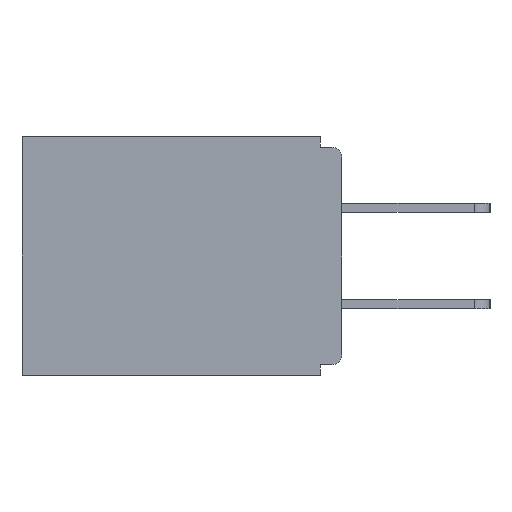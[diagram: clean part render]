
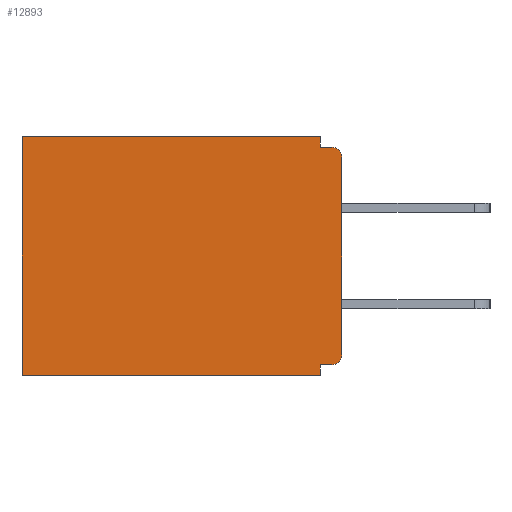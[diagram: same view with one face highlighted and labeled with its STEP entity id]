
A CAD part, left-side view. The second image highlights one B-rep face of the part: STEP entity #12893.
In plain terms, the highlighted planar face has unit normal (-1, 0, 0).
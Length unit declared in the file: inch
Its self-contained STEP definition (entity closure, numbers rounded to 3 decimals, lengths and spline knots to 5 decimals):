
#39 = LINE ( 'NONE', #16850, #4491 ) ;
#577 = EDGE_LOOP ( 'NONE', ( #16964, #21530, #7711, #17324, #13636, #9367, #11349, #9855, #5133, #16486 ) ) ;
#677 = VECTOR ( 'NONE', #12120, 39.37008 ) ;
#1747 = CARTESIAN_POINT ( 'NONE',  ( 0.298, 0., -0.343 ) ) ;
#2031 = DIRECTION ( 'NONE',  ( 0., 0., -1. ) ) ;
#3687 = DIRECTION ( 'NONE',  ( -1., 0., 0. ) ) ;
#3743 = DIRECTION ( 'NONE',  ( 0., 1., 0. ) ) ;
#4325 = LINE ( 'NONE', #12921, #9213 ) ;
#4491 = VECTOR ( 'NONE', #19099, 39.37008 ) ;
#4637 = CARTESIAN_POINT ( 'NONE',  ( 0.298, 0.46, 0. ) ) ;
#5065 = VERTEX_POINT ( 'NONE', #9523 ) ;
#5075 = DIRECTION ( 'NONE',  ( 0., 0., -1. ) ) ;
#5133 = ORIENTED_EDGE ( 'NONE', *, *, #8164, .T. ) ;
#5738 = CARTESIAN_POINT ( 'NONE',  ( 0.298, 0., 0. ) ) ;
#5801 = VERTEX_POINT ( 'NONE', #16505 ) ;
#6765 = DIRECTION ( 'NONE',  ( 0., 0., -1. ) ) ;
#6874 = AXIS2_PLACEMENT_3D ( 'NONE', #23758, #14232, #6765 ) ;
#7126 = CARTESIAN_POINT ( 'NONE',  ( 0.298, 0.015, -0.03 ) ) ;
#7220 = LINE ( 'NONE', #1747, #21941 ) ;
#7222 = FACE_OUTER_BOUND ( 'NONE', #577, .T. ) ;
#7273 = EDGE_CURVE ( 'NONE', #23118, #10167, #19019, .T. ) ;
#7279 = VECTOR ( 'NONE', #16930, 39.37008 ) ;
#7711 = ORIENTED_EDGE ( 'NONE', *, *, #9412, .F. ) ;
#7803 = CARTESIAN_POINT ( 'NONE',  ( 0.298, 0.031, -0.328 ) ) ;
#7809 = AXIS2_PLACEMENT_3D ( 'NONE', #7126, #11235, #5075 ) ;
#8164 = EDGE_CURVE ( 'NONE', #11813, #21252, #22765, .T. ) ;
#8405 = PLANE ( 'NONE',  #6874 ) ;
#8854 = DIRECTION ( 'NONE',  ( 0., 0., -1. ) ) ;
#9213 = VECTOR ( 'NONE', #8854, 39.37008 ) ;
#9367 = ORIENTED_EDGE ( 'NONE', *, *, #15010, .F. ) ;
#9412 = EDGE_CURVE ( 'NONE', #5801, #23985, #4325, .T. ) ;
#9523 = CARTESIAN_POINT ( 'NONE',  ( 0.298, 0., -0.03 ) ) ;
#9817 = DIRECTION ( 'NONE',  ( 0., 1., 0. ) ) ;
#9855 = ORIENTED_EDGE ( 'NONE', *, *, #14461, .F. ) ;
#10167 = VERTEX_POINT ( 'NONE', #11568 ) ;
#10659 = VECTOR ( 'NONE', #9817, 39.37008 ) ;
#10799 = EDGE_CURVE ( 'NONE', #5801, #23271, #22917, .T. ) ;
#10872 = AXIS2_PLACEMENT_3D ( 'NONE', #13351, #3687, #2031 ) ;
#11235 = DIRECTION ( 'NONE',  ( -1., 0., 0. ) ) ;
#11349 = ORIENTED_EDGE ( 'NONE', *, *, #7273, .F. ) ;
#11435 = CARTESIAN_POINT ( 'NONE',  ( 0.298, 0., -0.015 ) ) ;
#11568 = CARTESIAN_POINT ( 'NONE',  ( 0.298, 0.031, -0.343 ) ) ;
#11813 = VERTEX_POINT ( 'NONE', #16316 ) ;
#11872 = LINE ( 'NONE', #16394, #17180 ) ;
#11960 = EDGE_CURVE ( 'NONE', #23271, #18347, #11872, .T. ) ;
#12120 = DIRECTION ( 'NONE',  ( 0., 0., -1. ) ) ;
#12297 = CARTESIAN_POINT ( 'NONE',  ( 0.298, 0.46, -0.343 ) ) ;
#12352 = CARTESIAN_POINT ( 'NONE',  ( 0.298, 0., -0.313 ) ) ;
#12893 = ADVANCED_FACE ( 'NONE', ( #7222 ), #8405, .F. ) ;
#12921 = CARTESIAN_POINT ( 'NONE',  ( 0.298, 0.031, -0.343 ) ) ;
#13351 = CARTESIAN_POINT ( 'NONE',  ( 0.298, 0.015, -0.313 ) ) ;
#13636 = ORIENTED_EDGE ( 'NONE', *, *, #11960, .T. ) ;
#14063 = CARTESIAN_POINT ( 'NONE',  ( 0.298, 0.015, -0.015 ) ) ;
#14203 = CIRCLE ( 'NONE', #7809, 0.015 ) ;
#14232 = DIRECTION ( 'NONE',  ( 1., 0., 0. ) ) ;
#14461 = EDGE_CURVE ( 'NONE', #11813, #23118, #39, .T. ) ;
#15010 = EDGE_CURVE ( 'NONE', #10167, #18347, #7220, .T. ) ;
#15474 = DIRECTION ( 'NONE',  ( 0., 0., -1. ) ) ;
#15526 = VECTOR ( 'NONE', #17205, 39.37008 ) ;
#16316 = CARTESIAN_POINT ( 'NONE',  ( 0.298, 0.015, -0.328 ) ) ;
#16394 = CARTESIAN_POINT ( 'NONE',  ( 0.298, 0.46, 0. ) ) ;
#16486 = ORIENTED_EDGE ( 'NONE', *, *, #18054, .F. ) ;
#16505 = CARTESIAN_POINT ( 'NONE',  ( 0.298, 0.031, 0. ) ) ;
#16645 = LINE ( 'NONE', #11435, #7279 ) ;
#16707 = LINE ( 'NONE', #5738, #15526 ) ;
#16850 = CARTESIAN_POINT ( 'NONE',  ( 0.298, 0., -0.328 ) ) ;
#16930 = DIRECTION ( 'NONE',  ( 0., -1., 0. ) ) ;
#16964 = ORIENTED_EDGE ( 'NONE', *, *, #19788, .T. ) ;
#17180 = VECTOR ( 'NONE', #15474, 39.37008 ) ;
#17205 = DIRECTION ( 'NONE',  ( 0., 0., -1. ) ) ;
#17324 = ORIENTED_EDGE ( 'NONE', *, *, #10799, .T. ) ;
#17508 = CARTESIAN_POINT ( 'NONE',  ( 0.298, 0., 0. ) ) ;
#18054 = EDGE_CURVE ( 'NONE', #5065, #21252, #16707, .T. ) ;
#18347 = VERTEX_POINT ( 'NONE', #12297 ) ;
#18658 = VERTEX_POINT ( 'NONE', #14063 ) ;
#19019 = LINE ( 'NONE', #19918, #677 ) ;
#19099 = DIRECTION ( 'NONE',  ( 0., 1., 0. ) ) ;
#19276 = EDGE_CURVE ( 'NONE', #23985, #18658, #16645, .T. ) ;
#19788 = EDGE_CURVE ( 'NONE', #5065, #18658, #14203, .T. ) ;
#19918 = CARTESIAN_POINT ( 'NONE',  ( 0.298, 0.031, -0.343 ) ) ;
#21252 = VERTEX_POINT ( 'NONE', #12352 ) ;
#21530 = ORIENTED_EDGE ( 'NONE', *, *, #19276, .F. ) ;
#21941 = VECTOR ( 'NONE', #3743, 39.37008 ) ;
#22765 = CIRCLE ( 'NONE', #10872, 0.015 ) ;
#22917 = LINE ( 'NONE', #17508, #10659 ) ;
#23118 = VERTEX_POINT ( 'NONE', #7803 ) ;
#23271 = VERTEX_POINT ( 'NONE', #4637 ) ;
#23758 = CARTESIAN_POINT ( 'NONE',  ( 0.298, 0., 0. ) ) ;
#23797 = CARTESIAN_POINT ( 'NONE',  ( 0.298, 0.031, -0.015 ) ) ;
#23985 = VERTEX_POINT ( 'NONE', #23797 ) ;
